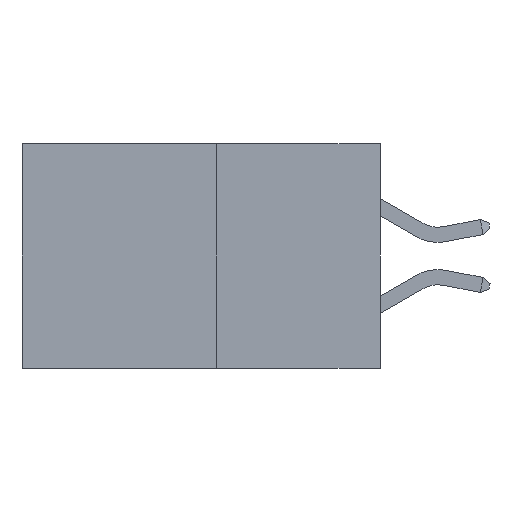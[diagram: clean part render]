
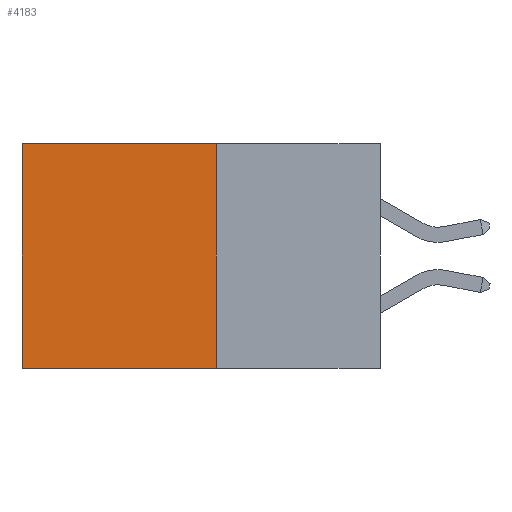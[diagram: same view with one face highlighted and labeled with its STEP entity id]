
A CAD part, left-side view. The second image highlights one B-rep face of the part: STEP entity #4183.
In plain terms, the highlighted planar face has unit normal (-1, 0, 0).
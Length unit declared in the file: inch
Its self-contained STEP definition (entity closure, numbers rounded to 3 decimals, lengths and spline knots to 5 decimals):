
#195 = DIRECTION ( 'NONE',  ( 0., 1., 0. ) ) ;
#1376 = CARTESIAN_POINT ( 'NONE',  ( 0.277, 0.59, -0.37 ) ) ;
#2201 = VECTOR ( 'NONE', #195, 39.37008 ) ;
#3051 = ORIENTED_EDGE ( 'NONE', *, *, #9959, .T. ) ;
#3446 = DIRECTION ( 'NONE',  ( 0., 1., 0. ) ) ;
#3876 = LINE ( 'NONE', #12471, #7831 ) ;
#4183 = ADVANCED_FACE ( 'NONE', ( #13749 ), #13238, .F. ) ;
#6311 = EDGE_CURVE ( 'NONE', #13169, #10599, #12313, .T. ) ;
#6814 = DIRECTION ( 'NONE',  ( 1., 0., 0. ) ) ;
#7831 = VECTOR ( 'NONE', #16785, 39.37008 ) ;
#7977 = VECTOR ( 'NONE', #14300, 39.37008 ) ;
#8329 = CARTESIAN_POINT ( 'NONE',  ( 0.277, 0.27, -0.37 ) ) ;
#8649 = DIRECTION ( 'NONE',  ( 0., 0., -1. ) ) ;
#8661 = ORIENTED_EDGE ( 'NONE', *, *, #6311, .F. ) ;
#9217 = LINE ( 'NONE', #13762, #13118 ) ;
#9904 = EDGE_CURVE ( 'NONE', #10599, #16696, #9217, .T. ) ;
#9959 = EDGE_CURVE ( 'NONE', #16739, #16696, #3876, .T. ) ;
#10599 = VERTEX_POINT ( 'NONE', #12382 ) ;
#12313 = LINE ( 'NONE', #14341, #7977 ) ;
#12382 = CARTESIAN_POINT ( 'NONE',  ( 0.277, 0.27, -0.37 ) ) ;
#12471 = CARTESIAN_POINT ( 'NONE',  ( 0.277, 0.59, -0.37 ) ) ;
#13118 = VECTOR ( 'NONE', #3446, 39.37008 ) ;
#13169 = VERTEX_POINT ( 'NONE', #16711 ) ;
#13238 = PLANE ( 'NONE',  #17329 ) ;
#13241 = CARTESIAN_POINT ( 'NONE',  ( 0.277, 0.59, 0. ) ) ;
#13749 = FACE_OUTER_BOUND ( 'NONE', #15990, .T. ) ;
#13762 = CARTESIAN_POINT ( 'NONE',  ( 0.277, 0.27, -0.37 ) ) ;
#14300 = DIRECTION ( 'NONE',  ( 0., 0., -1. ) ) ;
#14341 = CARTESIAN_POINT ( 'NONE',  ( 0.277, 0.27, -0.37 ) ) ;
#14370 = ORIENTED_EDGE ( 'NONE', *, *, #18087, .T. ) ;
#15032 = ORIENTED_EDGE ( 'NONE', *, *, #9904, .F. ) ;
#15990 = EDGE_LOOP ( 'NONE', ( #3051, #15032, #8661, #14370 ) ) ;
#16696 = VERTEX_POINT ( 'NONE', #1376 ) ;
#16711 = CARTESIAN_POINT ( 'NONE',  ( 0.277, 0.27, 0. ) ) ;
#16739 = VERTEX_POINT ( 'NONE', #13241 ) ;
#16785 = DIRECTION ( 'NONE',  ( 0., 0., -1. ) ) ;
#17329 = AXIS2_PLACEMENT_3D ( 'NONE', #8329, #6814, #8649 ) ;
#17728 = CARTESIAN_POINT ( 'NONE',  ( 0.277, 0.27, 0. ) ) ;
#17808 = LINE ( 'NONE', #17728, #2201 ) ;
#18087 = EDGE_CURVE ( 'NONE', #13169, #16739, #17808, .T. ) ;
